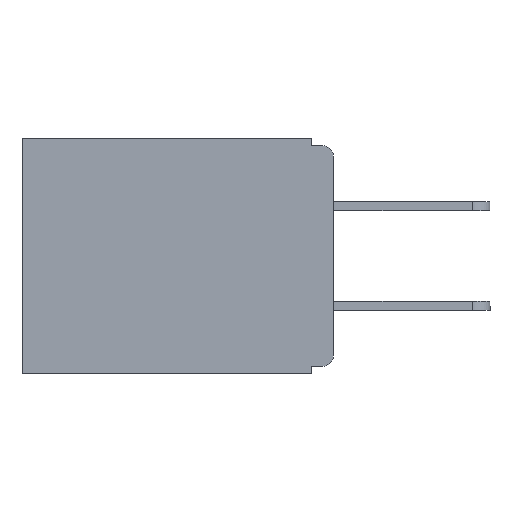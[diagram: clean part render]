
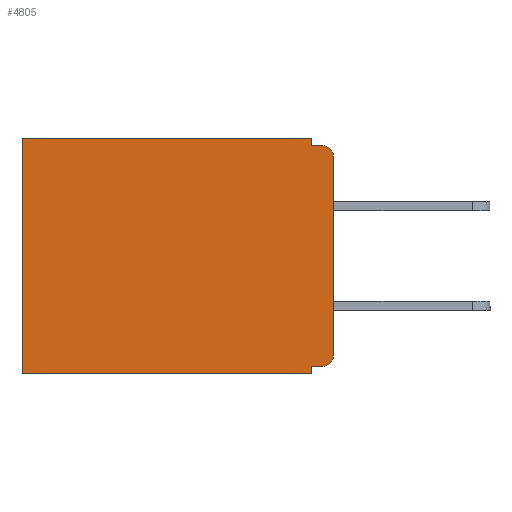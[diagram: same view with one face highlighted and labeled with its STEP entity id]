
A CAD part, left-side view. The second image highlights one B-rep face of the part: STEP entity #4805.
In plain terms, the highlighted planar face has unit normal (-1, 0, 0).
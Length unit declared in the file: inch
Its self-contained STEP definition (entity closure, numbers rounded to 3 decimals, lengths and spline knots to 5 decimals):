
#194 = CARTESIAN_POINT ( 'NONE',  ( 0.3, 0., -0.01 ) ) ;
#351 = CARTESIAN_POINT ( 'NONE',  ( 0.3, 0.031, 0. ) ) ;
#600 = ORIENTED_EDGE ( 'NONE', *, *, #11601, .T. ) ;
#1313 = DIRECTION ( 'NONE',  ( 0., 1., 0. ) ) ;
#1753 = DIRECTION ( 'NONE',  ( 0., 0., -1. ) ) ;
#1949 = VERTEX_POINT ( 'NONE', #6704 ) ;
#2738 = CARTESIAN_POINT ( 'NONE',  ( 0.3, 0.015, -0.025 ) ) ;
#2826 = VECTOR ( 'NONE', #1313, 39.37008 ) ;
#3172 = LINE ( 'NONE', #13761, #9901 ) ;
#3530 = ORIENTED_EDGE ( 'NONE', *, *, #14208, .T. ) ;
#3535 = VECTOR ( 'NONE', #9065, 39.37008 ) ;
#3618 = VERTEX_POINT ( 'NONE', #12372 ) ;
#3655 = ORIENTED_EDGE ( 'NONE', *, *, #16634, .T. ) ;
#3687 = VERTEX_POINT ( 'NONE', #9317 ) ;
#3731 = FACE_OUTER_BOUND ( 'NONE', #6884, .T. ) ;
#3979 = LINE ( 'NONE', #15556, #3535 ) ;
#4091 = DIRECTION ( 'NONE',  ( 0., 0., -1. ) ) ;
#4124 = EDGE_CURVE ( 'NONE', #3687, #9060, #10238, .T. ) ;
#4179 = VECTOR ( 'NONE', #17029, 39.37008 ) ;
#4467 = AXIS2_PLACEMENT_3D ( 'NONE', #7777, #11014, #10977 ) ;
#4795 = ORIENTED_EDGE ( 'NONE', *, *, #16859, .F. ) ;
#4805 = ADVANCED_FACE ( 'NONE', ( #3731 ), #15283, .F. ) ;
#4935 = CARTESIAN_POINT ( 'NONE',  ( 0.3, 0.015, -0.01 ) ) ;
#5024 = VERTEX_POINT ( 'NONE', #12880 ) ;
#5434 = CIRCLE ( 'NONE', #16425, 0.015 ) ;
#5443 = CARTESIAN_POINT ( 'NONE',  ( 0.3, 0.437, 0. ) ) ;
#5601 = DIRECTION ( 'NONE',  ( 0., 1., 0. ) ) ;
#5900 = ORIENTED_EDGE ( 'NONE', *, *, #11760, .T. ) ;
#6078 = EDGE_CURVE ( 'NONE', #1949, #9431, #16468, .T. ) ;
#6134 = ORIENTED_EDGE ( 'NONE', *, *, #8618, .F. ) ;
#6704 = CARTESIAN_POINT ( 'NONE',  ( 0.3, 0.031, -0.33 ) ) ;
#6884 = EDGE_LOOP ( 'NONE', ( #6134, #3530, #15159, #4795, #5900, #3655, #8068, #11062, #7202, #600 ) ) ;
#7202 = ORIENTED_EDGE ( 'NONE', *, *, #16760, .F. ) ;
#7684 = DIRECTION ( 'NONE',  ( -1., 0., 0. ) ) ;
#7777 = CARTESIAN_POINT ( 'NONE',  ( 0.3, 0., -0.33 ) ) ;
#7937 = VECTOR ( 'NONE', #9801, 39.37008 ) ;
#8068 = ORIENTED_EDGE ( 'NONE', *, *, #6078, .F. ) ;
#8206 = CARTESIAN_POINT ( 'NONE',  ( 0.3, 0., -0.305 ) ) ;
#8618 = EDGE_CURVE ( 'NONE', #11534, #16111, #3172, .T. ) ;
#8844 = CIRCLE ( 'NONE', #16985, 0.015 ) ;
#9060 = VERTEX_POINT ( 'NONE', #4935 ) ;
#9065 = DIRECTION ( 'NONE',  ( 0., 0., -1. ) ) ;
#9317 = CARTESIAN_POINT ( 'NONE',  ( 0.3, 0.031, -0.01 ) ) ;
#9431 = VERTEX_POINT ( 'NONE', #14817 ) ;
#9801 = DIRECTION ( 'NONE',  ( 0., 0., -1. ) ) ;
#9901 = VECTOR ( 'NONE', #1753, 39.37008 ) ;
#10238 = LINE ( 'NONE', #194, #16709 ) ;
#10364 = LINE ( 'NONE', #17116, #2826 ) ;
#10606 = CARTESIAN_POINT ( 'NONE',  ( 0.3, 0.437, -0.33 ) ) ;
#10977 = DIRECTION ( 'NONE',  ( 0., 0., -1. ) ) ;
#11014 = DIRECTION ( 'NONE',  ( 1., 0., 0. ) ) ;
#11062 = ORIENTED_EDGE ( 'NONE', *, *, #16011, .F. ) ;
#11534 = VERTEX_POINT ( 'NONE', #14019 ) ;
#11601 = EDGE_CURVE ( 'NONE', #5024, #16111, #5434, .T. ) ;
#11677 = LINE ( 'NONE', #10606, #4179 ) ;
#11760 = EDGE_CURVE ( 'NONE', #3618, #14202, #10364, .T. ) ;
#12074 = DIRECTION ( 'NONE',  ( -1., 0., 0. ) ) ;
#12372 = CARTESIAN_POINT ( 'NONE',  ( 0.3, 0.031, 0. ) ) ;
#12467 = DIRECTION ( 'NONE',  ( 0., -1., 0. ) ) ;
#12880 = CARTESIAN_POINT ( 'NONE',  ( 0.3, 0.015, -0.32 ) ) ;
#13523 = VECTOR ( 'NONE', #5601, 39.37008 ) ;
#13761 = CARTESIAN_POINT ( 'NONE',  ( 0.3, 0., -0.33 ) ) ;
#14019 = CARTESIAN_POINT ( 'NONE',  ( 0.3, 0., -0.025 ) ) ;
#14029 = DIRECTION ( 'NONE',  ( 0., 1., 0. ) ) ;
#14202 = VERTEX_POINT ( 'NONE', #5443 ) ;
#14208 = EDGE_CURVE ( 'NONE', #11534, #9060, #8844, .T. ) ;
#14449 = CARTESIAN_POINT ( 'NONE',  ( 0.3, 0., -0.33 ) ) ;
#14776 = CARTESIAN_POINT ( 'NONE',  ( 0.3, 0., -0.32 ) ) ;
#14817 = CARTESIAN_POINT ( 'NONE',  ( 0.3, 0.437, -0.33 ) ) ;
#14901 = VECTOR ( 'NONE', #14029, 39.37008 ) ;
#14917 = LINE ( 'NONE', #351, #7937 ) ;
#15159 = ORIENTED_EDGE ( 'NONE', *, *, #4124, .F. ) ;
#15218 = CARTESIAN_POINT ( 'NONE',  ( 0.3, 0.031, -0.32 ) ) ;
#15283 = PLANE ( 'NONE',  #4467 ) ;
#15520 = CARTESIAN_POINT ( 'NONE',  ( 0.3, 0.015, -0.305 ) ) ;
#15556 = CARTESIAN_POINT ( 'NONE',  ( 0.3, 0.031, -0.33 ) ) ;
#16011 = EDGE_CURVE ( 'NONE', #16336, #1949, #3979, .T. ) ;
#16102 = LINE ( 'NONE', #14776, #13523 ) ;
#16111 = VERTEX_POINT ( 'NONE', #8206 ) ;
#16336 = VERTEX_POINT ( 'NONE', #15218 ) ;
#16425 = AXIS2_PLACEMENT_3D ( 'NONE', #15520, #7684, #16777 ) ;
#16468 = LINE ( 'NONE', #14449, #14901 ) ;
#16634 = EDGE_CURVE ( 'NONE', #14202, #9431, #11677, .T. ) ;
#16709 = VECTOR ( 'NONE', #12467, 39.37008 ) ;
#16760 = EDGE_CURVE ( 'NONE', #5024, #16336, #16102, .T. ) ;
#16777 = DIRECTION ( 'NONE',  ( 0., 0., -1. ) ) ;
#16859 = EDGE_CURVE ( 'NONE', #3618, #3687, #14917, .T. ) ;
#16985 = AXIS2_PLACEMENT_3D ( 'NONE', #2738, #12074, #4091 ) ;
#17029 = DIRECTION ( 'NONE',  ( 0., 0., -1. ) ) ;
#17116 = CARTESIAN_POINT ( 'NONE',  ( 0.3, 0., 0. ) ) ;
